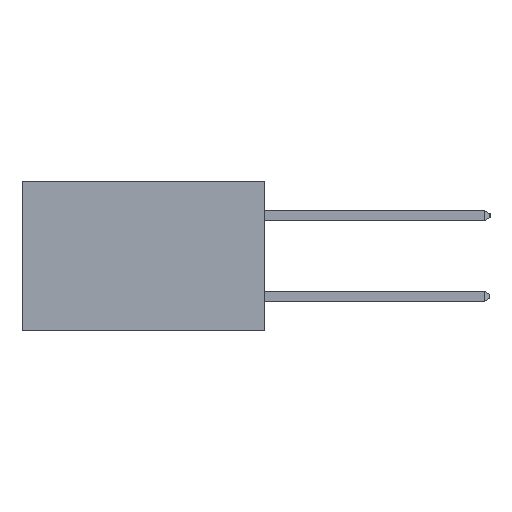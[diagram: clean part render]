
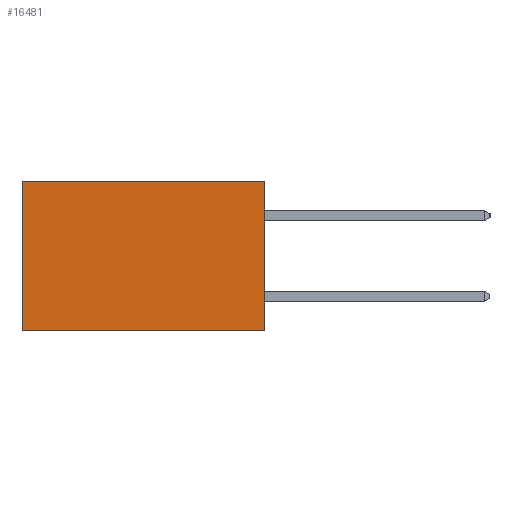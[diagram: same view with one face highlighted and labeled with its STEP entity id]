
A CAD part, left-side view. The second image highlights one B-rep face of the part: STEP entity #16481.
In plain terms, the highlighted planar face has unit normal (-1, 0, 0).
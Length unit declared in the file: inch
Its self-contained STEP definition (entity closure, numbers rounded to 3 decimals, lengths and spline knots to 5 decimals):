
#727 = CARTESIAN_POINT ( 'NONE',  ( 0.2615, 0.6, -0.37 ) ) ;
#729 = VERTEX_POINT ( 'NONE', #25481 ) ;
#1448 = LINE ( 'NONE', #9269, #7933 ) ;
#1854 = DIRECTION ( 'NONE',  ( 0., 1., 0. ) ) ;
#2145 = DIRECTION ( 'NONE',  ( 0., 0., -1. ) ) ;
#2342 = EDGE_CURVE ( 'NONE', #11987, #23234, #1448, .T. ) ;
#3004 = DIRECTION ( 'NONE',  ( 0., 0., -1. ) ) ;
#3610 = AXIS2_PLACEMENT_3D ( 'NONE', #20948, #22793, #3004 ) ;
#7933 = VECTOR ( 'NONE', #21106, 39.37008 ) ;
#8150 = LINE ( 'NONE', #13979, #21692 ) ;
#8292 = VECTOR ( 'NONE', #1854, 39.37008 ) ;
#9269 = CARTESIAN_POINT ( 'NONE',  ( 0.2615, 0., 0. ) ) ;
#9973 = CARTESIAN_POINT ( 'NONE',  ( 0.2615, 0., -0.37 ) ) ;
#10234 = CARTESIAN_POINT ( 'NONE',  ( 0.2615, 0., 0. ) ) ;
#11987 = VERTEX_POINT ( 'NONE', #10234 ) ;
#12140 = EDGE_CURVE ( 'NONE', #729, #20700, #21649, .T. ) ;
#13683 = VECTOR ( 'NONE', #2145, 39.37008 ) ;
#13979 = CARTESIAN_POINT ( 'NONE',  ( 0.2615, 0.6, -0.37 ) ) ;
#14466 = PLANE ( 'NONE',  #3610 ) ;
#16481 = ADVANCED_FACE ( 'NONE', ( #16780 ), #14466, .F. ) ;
#16659 = CARTESIAN_POINT ( 'NONE',  ( 0.2615, 0.6, 0. ) ) ;
#16780 = FACE_OUTER_BOUND ( 'NONE', #17848, .T. ) ;
#17615 = CARTESIAN_POINT ( 'NONE',  ( 0.2615, 0., -0.37 ) ) ;
#17848 = EDGE_LOOP ( 'NONE', ( #21947, #19047, #21421, #25041 ) ) ;
#19047 = ORIENTED_EDGE ( 'NONE', *, *, #12140, .F. ) ;
#19581 = DIRECTION ( 'NONE',  ( 0., 0., -1. ) ) ;
#19981 = LINE ( 'NONE', #9973, #13683 ) ;
#20700 = VERTEX_POINT ( 'NONE', #727 ) ;
#20948 = CARTESIAN_POINT ( 'NONE',  ( 0.2615, 0., -0.37 ) ) ;
#21106 = DIRECTION ( 'NONE',  ( 0., 1., 0. ) ) ;
#21421 = ORIENTED_EDGE ( 'NONE', *, *, #22190, .F. ) ;
#21649 = LINE ( 'NONE', #17615, #8292 ) ;
#21692 = VECTOR ( 'NONE', #19581, 39.37008 ) ;
#21947 = ORIENTED_EDGE ( 'NONE', *, *, #25612, .T. ) ;
#22190 = EDGE_CURVE ( 'NONE', #11987, #729, #19981, .T. ) ;
#22793 = DIRECTION ( 'NONE',  ( 1., 0., 0. ) ) ;
#23234 = VERTEX_POINT ( 'NONE', #16659 ) ;
#25041 = ORIENTED_EDGE ( 'NONE', *, *, #2342, .T. ) ;
#25481 = CARTESIAN_POINT ( 'NONE',  ( 0.2615, 0., -0.37 ) ) ;
#25612 = EDGE_CURVE ( 'NONE', #23234, #20700, #8150, .T. ) ;
